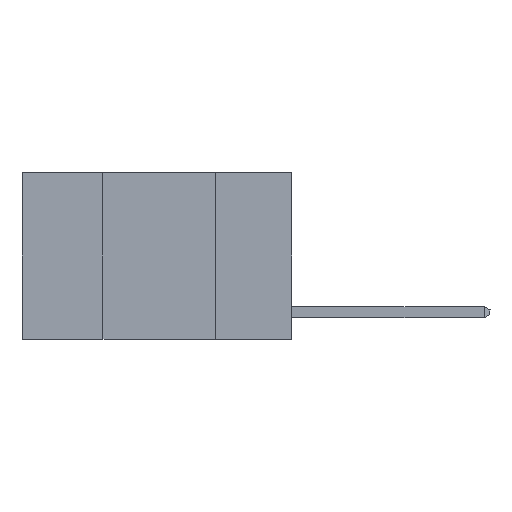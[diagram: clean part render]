
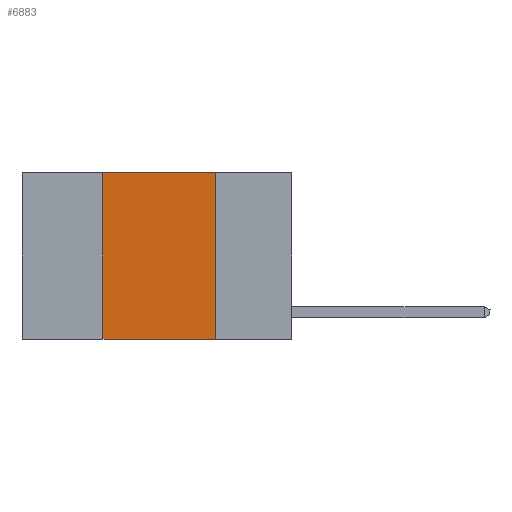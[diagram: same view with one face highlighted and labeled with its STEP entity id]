
A CAD part, left-side view. The second image highlights one B-rep face of the part: STEP entity #6883.
In plain terms, the highlighted planar face has unit normal (-1, 0, 0).
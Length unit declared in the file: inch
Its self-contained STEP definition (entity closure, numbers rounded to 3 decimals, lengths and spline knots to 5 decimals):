
#220 = EDGE_CURVE ( 'NONE', #9862, #6041, #12463, .T. ) ;
#363 = VECTOR ( 'NONE', #15080, 39.37008 ) ;
#472 = DIRECTION ( 'NONE',  ( 1., 0., 0. ) ) ;
#552 = LINE ( 'NONE', #16605, #16531 ) ;
#1809 = CARTESIAN_POINT ( 'NONE',  ( 0., 0.17, 0. ) ) ;
#1817 = ORIENTED_EDGE ( 'NONE', *, *, #15018, .F. ) ;
#3002 = LINE ( 'NONE', #11344, #12261 ) ;
#3752 = CARTESIAN_POINT ( 'NONE',  ( 0., 0.17, 0. ) ) ;
#4095 = AXIS2_PLACEMENT_3D ( 'NONE', #14106, #472, #5958 ) ;
#5958 = DIRECTION ( 'NONE',  ( 0., 0., -1. ) ) ;
#6041 = VERTEX_POINT ( 'NONE', #11988 ) ;
#6195 = CARTESIAN_POINT ( 'NONE',  ( 0., 0.42, -0.37 ) ) ;
#6883 = ADVANCED_FACE ( 'NONE', ( #7284 ), #8627, .F. ) ;
#7284 = FACE_OUTER_BOUND ( 'NONE', #15394, .T. ) ;
#8349 = CARTESIAN_POINT ( 'NONE',  ( 0., 0.6, -0.37 ) ) ;
#8488 = DIRECTION ( 'NONE',  ( 0., -1., 0. ) ) ;
#8627 = PLANE ( 'NONE',  #4095 ) ;
#9054 = ORIENTED_EDGE ( 'NONE', *, *, #13479, .F. ) ;
#9862 = VERTEX_POINT ( 'NONE', #6195 ) ;
#9918 = VERTEX_POINT ( 'NONE', #11541 ) ;
#11091 = ORIENTED_EDGE ( 'NONE', *, *, #220, .T. ) ;
#11344 = CARTESIAN_POINT ( 'NONE',  ( 0., 0.6, 0. ) ) ;
#11541 = CARTESIAN_POINT ( 'NONE',  ( 0., 0.42, 0. ) ) ;
#11988 = CARTESIAN_POINT ( 'NONE',  ( 0., 0.17, -0.37 ) ) ;
#12261 = VECTOR ( 'NONE', #8488, 39.37008 ) ;
#12463 = LINE ( 'NONE', #8349, #363 ) ;
#13479 = EDGE_CURVE ( 'NONE', #9862, #9918, #552, .T. ) ;
#13918 = DIRECTION ( 'NONE',  ( 0., 0., 1. ) ) ;
#14106 = CARTESIAN_POINT ( 'NONE',  ( 0., 0.6, 0. ) ) ;
#14123 = ORIENTED_EDGE ( 'NONE', *, *, #14870, .F. ) ;
#14336 = DIRECTION ( 'NONE',  ( 0., 0., -1. ) ) ;
#14567 = VECTOR ( 'NONE', #14336, 39.37008 ) ;
#14870 = EDGE_CURVE ( 'NONE', #17138, #6041, #16047, .T. ) ;
#15018 = EDGE_CURVE ( 'NONE', #9918, #17138, #3002, .T. ) ;
#15080 = DIRECTION ( 'NONE',  ( 0., -1., 0. ) ) ;
#15394 = EDGE_LOOP ( 'NONE', ( #14123, #1817, #9054, #11091 ) ) ;
#16047 = LINE ( 'NONE', #3752, #14567 ) ;
#16531 = VECTOR ( 'NONE', #13918, 39.37008 ) ;
#16605 = CARTESIAN_POINT ( 'NONE',  ( 0., 0.42, 0. ) ) ;
#17138 = VERTEX_POINT ( 'NONE', #1809 ) ;
